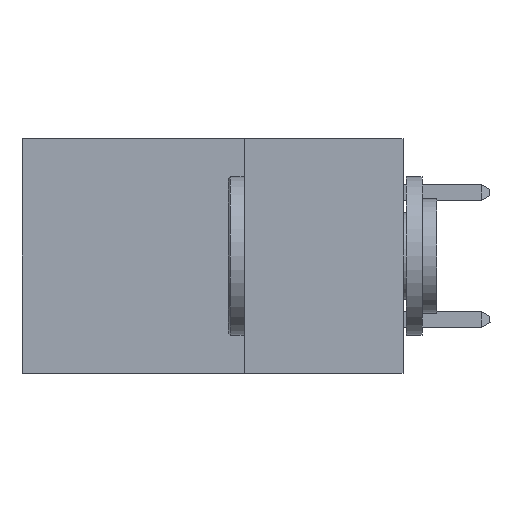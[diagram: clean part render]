
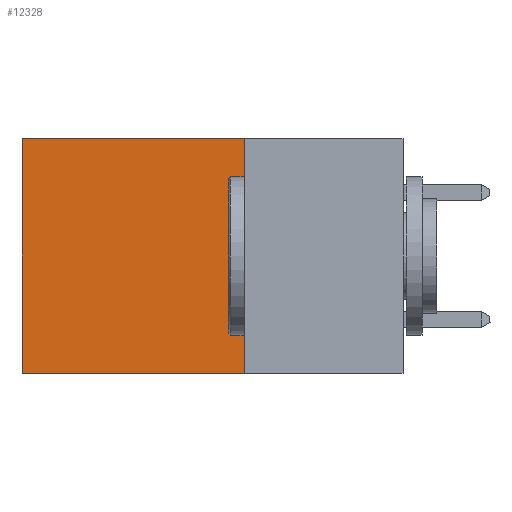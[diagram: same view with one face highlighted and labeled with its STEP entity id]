
A CAD part, left-side view. The second image highlights one B-rep face of the part: STEP entity #12328.
In plain terms, the highlighted planar face has unit normal (-1, 0, 0).
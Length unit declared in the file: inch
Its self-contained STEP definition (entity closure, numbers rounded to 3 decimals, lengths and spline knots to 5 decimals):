
#1815 = PLANE ( 'NONE',  #10222 ) ;
#2647 = EDGE_CURVE ( 'NONE', #4819, #22315, #10450, .T. ) ;
#3209 = EDGE_LOOP ( 'NONE', ( #8061, #20884, #4226, #13132 ) ) ;
#4226 = ORIENTED_EDGE ( 'NONE', *, *, #19669, .F. ) ;
#4819 = VERTEX_POINT ( 'NONE', #7035 ) ;
#4931 = VERTEX_POINT ( 'NONE', #21109 ) ;
#5379 = EDGE_CURVE ( 'NONE', #13861, #22315, #14966, .T. ) ;
#5430 = DIRECTION ( 'NONE',  ( 1., 0., 0. ) ) ;
#5618 = DIRECTION ( 'NONE',  ( 0., 0., -1. ) ) ;
#6340 = FACE_OUTER_BOUND ( 'NONE', #3209, .T. ) ;
#6749 = DIRECTION ( 'NONE',  ( 0., 1., 0. ) ) ;
#6879 = VECTOR ( 'NONE', #14048, 39.37008 ) ;
#7035 = CARTESIAN_POINT ( 'NONE',  ( 0.2875, 0.25, -0.37 ) ) ;
#7139 = CARTESIAN_POINT ( 'NONE',  ( 0.2875, 0.25, -0.37 ) ) ;
#7140 = CARTESIAN_POINT ( 'NONE',  ( 0.2875, 0.25, 0. ) ) ;
#7315 = CARTESIAN_POINT ( 'NONE',  ( 0.2875, 0.25, 0. ) ) ;
#8061 = ORIENTED_EDGE ( 'NONE', *, *, #5379, .T. ) ;
#9328 = VECTOR ( 'NONE', #6749, 39.37008 ) ;
#10222 = AXIS2_PLACEMENT_3D ( 'NONE', #15795, #5430, #17565 ) ;
#10347 = VECTOR ( 'NONE', #20584, 39.37008 ) ;
#10450 = LINE ( 'NONE', #7139, #9328 ) ;
#12328 = ADVANCED_FACE ( 'NONE', ( #6340 ), #1815, .F. ) ;
#12333 = EDGE_CURVE ( 'NONE', #4931, #13861, #20097, .T. ) ;
#13132 = ORIENTED_EDGE ( 'NONE', *, *, #12333, .T. ) ;
#13230 = CARTESIAN_POINT ( 'NONE',  ( 0.2875, 0.6, 0. ) ) ;
#13861 = VERTEX_POINT ( 'NONE', #13230 ) ;
#14048 = DIRECTION ( 'NONE',  ( 0., 1., 0. ) ) ;
#14946 = LINE ( 'NONE', #7315, #19015 ) ;
#14966 = LINE ( 'NONE', #17220, #10347 ) ;
#15305 = CARTESIAN_POINT ( 'NONE',  ( 0.2875, 0.6, -0.37 ) ) ;
#15795 = CARTESIAN_POINT ( 'NONE',  ( 0.2875, 0.25, 0. ) ) ;
#17220 = CARTESIAN_POINT ( 'NONE',  ( 0.2875, 0.6, 0. ) ) ;
#17565 = DIRECTION ( 'NONE',  ( 0., 0., -1. ) ) ;
#19015 = VECTOR ( 'NONE', #5618, 39.37008 ) ;
#19669 = EDGE_CURVE ( 'NONE', #4931, #4819, #14946, .T. ) ;
#20097 = LINE ( 'NONE', #7140, #6879 ) ;
#20584 = DIRECTION ( 'NONE',  ( 0., 0., -1. ) ) ;
#20884 = ORIENTED_EDGE ( 'NONE', *, *, #2647, .F. ) ;
#21109 = CARTESIAN_POINT ( 'NONE',  ( 0.2875, 0.25, 0. ) ) ;
#22315 = VERTEX_POINT ( 'NONE', #15305 ) ;
